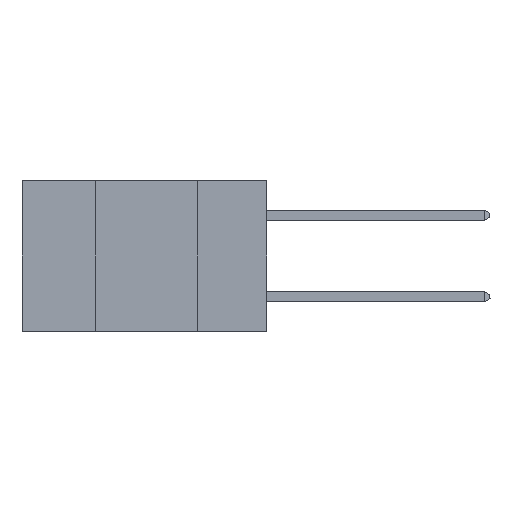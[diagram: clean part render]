
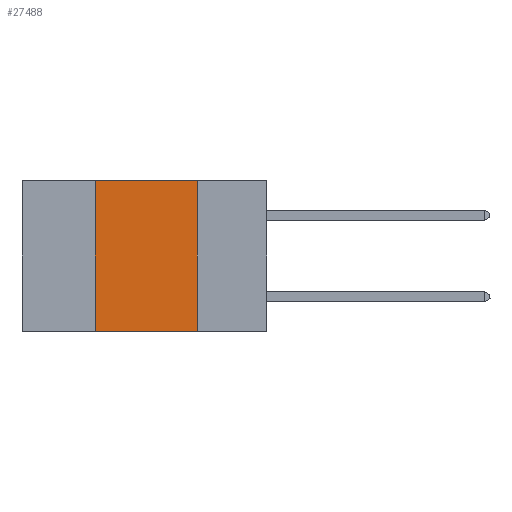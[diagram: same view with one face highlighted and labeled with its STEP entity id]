
A CAD part, left-side view. The second image highlights one B-rep face of the part: STEP entity #27488.
In plain terms, the highlighted planar face has unit normal (-1, 0, 0).
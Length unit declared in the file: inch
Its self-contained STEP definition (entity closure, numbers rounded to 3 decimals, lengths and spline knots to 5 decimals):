
#691 = CARTESIAN_POINT ( 'NONE',  ( 0., 0.6, 0. ) ) ;
#1049 = CARTESIAN_POINT ( 'NONE',  ( 0., 0.42, 0. ) ) ;
#1096 = CARTESIAN_POINT ( 'NONE',  ( 0., 0.17, 0. ) ) ;
#2347 = CARTESIAN_POINT ( 'NONE',  ( 0., 0.6, -0.37 ) ) ;
#4257 = EDGE_CURVE ( 'NONE', #11729, #15292, #25107, .T. ) ;
#4285 = CARTESIAN_POINT ( 'NONE',  ( 0., 0.42, 0. ) ) ;
#4410 = VECTOR ( 'NONE', #5105, 39.37008 ) ;
#4478 = ORIENTED_EDGE ( 'NONE', *, *, #25152, .T. ) ;
#5105 = DIRECTION ( 'NONE',  ( 0., -1., 0. ) ) ;
#5245 = VERTEX_POINT ( 'NONE', #1049 ) ;
#5965 = ORIENTED_EDGE ( 'NONE', *, *, #4257, .F. ) ;
#6006 = ORIENTED_EDGE ( 'NONE', *, *, #12192, .F. ) ;
#6602 = VECTOR ( 'NONE', #11583, 39.37008 ) ;
#7221 = ORIENTED_EDGE ( 'NONE', *, *, #13857, .F. ) ;
#8849 = DIRECTION ( 'NONE',  ( 0., 0., -1. ) ) ;
#11583 = DIRECTION ( 'NONE',  ( 0., 0., -1. ) ) ;
#11729 = VERTEX_POINT ( 'NONE', #12269 ) ;
#12192 = EDGE_CURVE ( 'NONE', #5245, #11729, #13994, .T. ) ;
#12269 = CARTESIAN_POINT ( 'NONE',  ( 0., 0.17, 0. ) ) ;
#12840 = CARTESIAN_POINT ( 'NONE',  ( 0., 0.17, -0.37 ) ) ;
#13622 = EDGE_LOOP ( 'NONE', ( #5965, #6006, #7221, #4478 ) ) ;
#13857 = EDGE_CURVE ( 'NONE', #14425, #5245, #24249, .T. ) ;
#13994 = LINE ( 'NONE', #691, #23004 ) ;
#14425 = VERTEX_POINT ( 'NONE', #27104 ) ;
#15067 = PLANE ( 'NONE',  #25200 ) ;
#15115 = DIRECTION ( 'NONE',  ( 0., 0., 1. ) ) ;
#15292 = VERTEX_POINT ( 'NONE', #12840 ) ;
#15863 = LINE ( 'NONE', #2347, #4410 ) ;
#16096 = FACE_OUTER_BOUND ( 'NONE', #13622, .T. ) ;
#18875 = VECTOR ( 'NONE', #15115, 39.37008 ) ;
#21503 = DIRECTION ( 'NONE',  ( 1., 0., 0. ) ) ;
#22737 = DIRECTION ( 'NONE',  ( 0., -1., 0. ) ) ;
#23004 = VECTOR ( 'NONE', #22737, 39.37008 ) ;
#23759 = CARTESIAN_POINT ( 'NONE',  ( 0., 0.6, 0. ) ) ;
#24249 = LINE ( 'NONE', #4285, #18875 ) ;
#25107 = LINE ( 'NONE', #1096, #6602 ) ;
#25152 = EDGE_CURVE ( 'NONE', #14425, #15292, #15863, .T. ) ;
#25200 = AXIS2_PLACEMENT_3D ( 'NONE', #23759, #21503, #8849 ) ;
#27104 = CARTESIAN_POINT ( 'NONE',  ( 0., 0.42, -0.37 ) ) ;
#27488 = ADVANCED_FACE ( 'NONE', ( #16096 ), #15067, .F. ) ;
